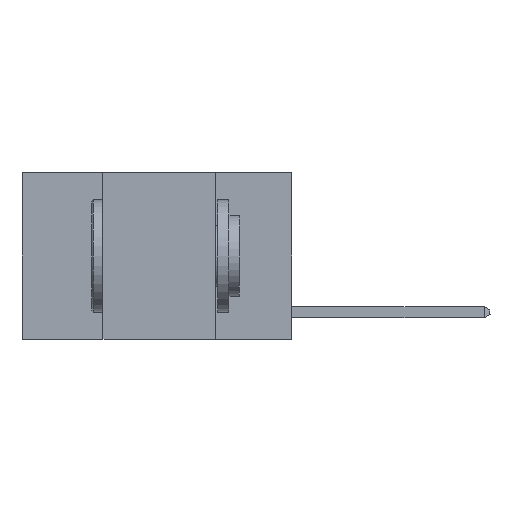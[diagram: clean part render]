
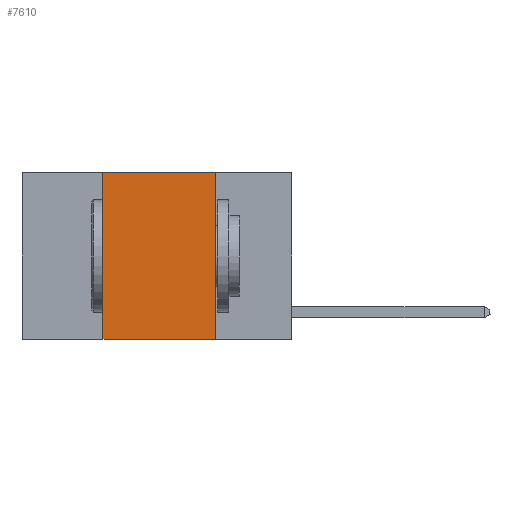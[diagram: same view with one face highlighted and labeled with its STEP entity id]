
A CAD part, left-side view. The second image highlights one B-rep face of the part: STEP entity #7610.
In plain terms, the highlighted planar face has unit normal (-1, 0, 0).
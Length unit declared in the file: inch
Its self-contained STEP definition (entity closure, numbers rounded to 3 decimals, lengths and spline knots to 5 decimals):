
#270 = CARTESIAN_POINT ( 'NONE',  ( 0., 0.6, 0. ) ) ;
#586 = PLANE ( 'NONE',  #16673 ) ;
#604 = VECTOR ( 'NONE', #10976, 39.37008 ) ;
#2492 = EDGE_CURVE ( 'NONE', #16308, #20350, #15756, .T. ) ;
#2779 = CARTESIAN_POINT ( 'NONE',  ( 0., 0.42, 0. ) ) ;
#4856 = LINE ( 'NONE', #6234, #11809 ) ;
#5440 = CARTESIAN_POINT ( 'NONE',  ( 0., 0.6, 0. ) ) ;
#5477 = DIRECTION ( 'NONE',  ( 0., 0., 1. ) ) ;
#5795 = ORIENTED_EDGE ( 'NONE', *, *, #12697, .F. ) ;
#6090 = CARTESIAN_POINT ( 'NONE',  ( 0., 0.17, 0. ) ) ;
#6234 = CARTESIAN_POINT ( 'NONE',  ( 0., 0.6, -0.37 ) ) ;
#6412 = ORIENTED_EDGE ( 'NONE', *, *, #2492, .F. ) ;
#6736 = DIRECTION ( 'NONE',  ( 1., 0., 0. ) ) ;
#7610 = ADVANCED_FACE ( 'NONE', ( #15241 ), #586, .F. ) ;
#8009 = CARTESIAN_POINT ( 'NONE',  ( 0., 0.17, 0. ) ) ;
#8369 = VECTOR ( 'NONE', #13427, 39.37008 ) ;
#10134 = DIRECTION ( 'NONE',  ( 0., 0., -1. ) ) ;
#10583 = ORIENTED_EDGE ( 'NONE', *, *, #20036, .T. ) ;
#10895 = CARTESIAN_POINT ( 'NONE',  ( 0., 0.17, -0.37 ) ) ;
#10976 = DIRECTION ( 'NONE',  ( 0., 0., -1. ) ) ;
#11809 = VECTOR ( 'NONE', #16326, 39.37008 ) ;
#12697 = EDGE_CURVE ( 'NONE', #17175, #16308, #16920, .T. ) ;
#13427 = DIRECTION ( 'NONE',  ( 0., -1., 0. ) ) ;
#13678 = LINE ( 'NONE', #13770, #13936 ) ;
#13770 = CARTESIAN_POINT ( 'NONE',  ( 0., 0.42, 0. ) ) ;
#13936 = VECTOR ( 'NONE', #5477, 39.37008 ) ;
#14324 = VERTEX_POINT ( 'NONE', #14550 ) ;
#14550 = CARTESIAN_POINT ( 'NONE',  ( 0., 0.42, -0.37 ) ) ;
#15241 = FACE_OUTER_BOUND ( 'NONE', #18926, .T. ) ;
#15756 = LINE ( 'NONE', #6090, #604 ) ;
#16222 = EDGE_CURVE ( 'NONE', #14324, #17175, #13678, .T. ) ;
#16308 = VERTEX_POINT ( 'NONE', #8009 ) ;
#16326 = DIRECTION ( 'NONE',  ( 0., -1., 0. ) ) ;
#16673 = AXIS2_PLACEMENT_3D ( 'NONE', #270, #6736, #10134 ) ;
#16920 = LINE ( 'NONE', #5440, #8369 ) ;
#17175 = VERTEX_POINT ( 'NONE', #2779 ) ;
#18926 = EDGE_LOOP ( 'NONE', ( #6412, #5795, #19213, #10583 ) ) ;
#19213 = ORIENTED_EDGE ( 'NONE', *, *, #16222, .F. ) ;
#20036 = EDGE_CURVE ( 'NONE', #14324, #20350, #4856, .T. ) ;
#20350 = VERTEX_POINT ( 'NONE', #10895 ) ;
